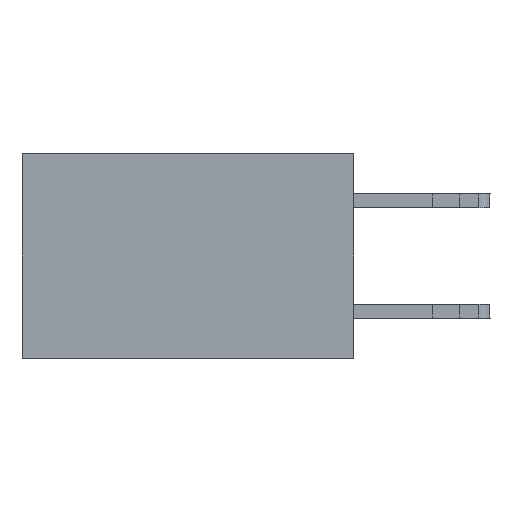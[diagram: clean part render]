
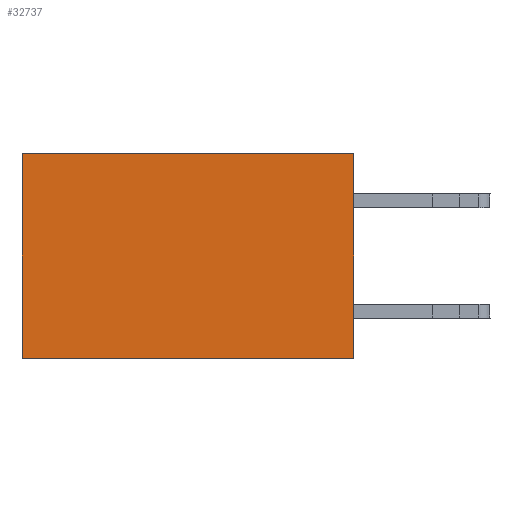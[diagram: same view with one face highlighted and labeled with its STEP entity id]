
A CAD part, left-side view. The second image highlights one B-rep face of the part: STEP entity #32737.
In plain terms, the highlighted planar face has unit normal (-1, 0, 0).
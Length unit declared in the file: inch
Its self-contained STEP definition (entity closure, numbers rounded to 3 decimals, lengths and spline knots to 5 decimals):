
#1080 = VERTEX_POINT ( 'NONE', #15323 ) ;
#1343 = CARTESIAN_POINT ( 'NONE',  ( 0.2875, 0., 0. ) ) ;
#2731 = LINE ( 'NONE', #1343, #19456 ) ;
#3647 = ORIENTED_EDGE ( 'NONE', *, *, #33575, .T. ) ;
#4345 = LINE ( 'NONE', #30931, #32164 ) ;
#5210 = DIRECTION ( 'NONE',  ( 0., 0., -1. ) ) ;
#6998 = CARTESIAN_POINT ( 'NONE',  ( 0.2875, 0., 0. ) ) ;
#7454 = VERTEX_POINT ( 'NONE', #14265 ) ;
#9291 = VECTOR ( 'NONE', #17194, 39.37008 ) ;
#11481 = DIRECTION ( 'NONE',  ( 1., 0., 0. ) ) ;
#14265 = CARTESIAN_POINT ( 'NONE',  ( 0.2875, 0., -0.37 ) ) ;
#15307 = ORIENTED_EDGE ( 'NONE', *, *, #21938, .T. ) ;
#15323 = CARTESIAN_POINT ( 'NONE',  ( 0.2875, 0.6, 0. ) ) ;
#15797 = FACE_OUTER_BOUND ( 'NONE', #20898, .T. ) ;
#16294 = VERTEX_POINT ( 'NONE', #23914 ) ;
#17194 = DIRECTION ( 'NONE',  ( 0., 0., -1. ) ) ;
#18246 = VERTEX_POINT ( 'NONE', #6998 ) ;
#18723 = LINE ( 'NONE', #24665, #9291 ) ;
#19456 = VECTOR ( 'NONE', #22324, 39.37008 ) ;
#20093 = ORIENTED_EDGE ( 'NONE', *, *, #26827, .F. ) ;
#20898 = EDGE_LOOP ( 'NONE', ( #15307, #20093, #32194, #3647 ) ) ;
#21159 = LINE ( 'NONE', #26202, #26852 ) ;
#21379 = CARTESIAN_POINT ( 'NONE',  ( 0.2875, 0., 0. ) ) ;
#21938 = EDGE_CURVE ( 'NONE', #1080, #16294, #21159, .T. ) ;
#22324 = DIRECTION ( 'NONE',  ( 0., 1., 0. ) ) ;
#23914 = CARTESIAN_POINT ( 'NONE',  ( 0.2875, 0.6, -0.37 ) ) ;
#24665 = CARTESIAN_POINT ( 'NONE',  ( 0.2875, 0., 0. ) ) ;
#25429 = EDGE_CURVE ( 'NONE', #18246, #7454, #18723, .T. ) ;
#26202 = CARTESIAN_POINT ( 'NONE',  ( 0.2875, 0.6, 0. ) ) ;
#26827 = EDGE_CURVE ( 'NONE', #7454, #16294, #4345, .T. ) ;
#26852 = VECTOR ( 'NONE', #5210, 39.37008 ) ;
#29148 = PLANE ( 'NONE',  #31129 ) ;
#29832 = DIRECTION ( 'NONE',  ( 0., 0., -1. ) ) ;
#30931 = CARTESIAN_POINT ( 'NONE',  ( 0.2875, 0., -0.37 ) ) ;
#31129 = AXIS2_PLACEMENT_3D ( 'NONE', #21379, #11481, #29832 ) ;
#32164 = VECTOR ( 'NONE', #33365, 39.37008 ) ;
#32194 = ORIENTED_EDGE ( 'NONE', *, *, #25429, .F. ) ;
#32737 = ADVANCED_FACE ( 'NONE', ( #15797 ), #29148, .F. ) ;
#33365 = DIRECTION ( 'NONE',  ( 0., 1., 0. ) ) ;
#33575 = EDGE_CURVE ( 'NONE', #18246, #1080, #2731, .T. ) ;
